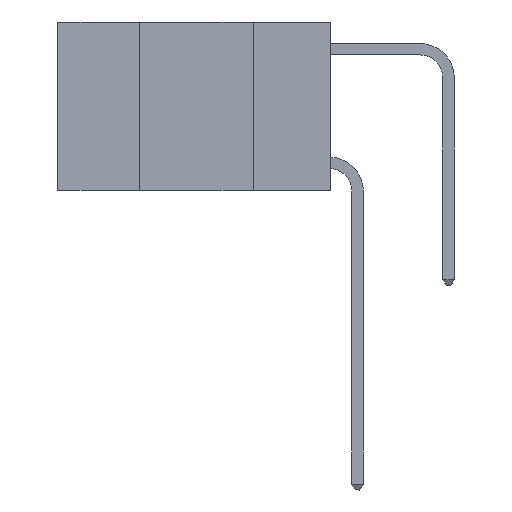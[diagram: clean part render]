
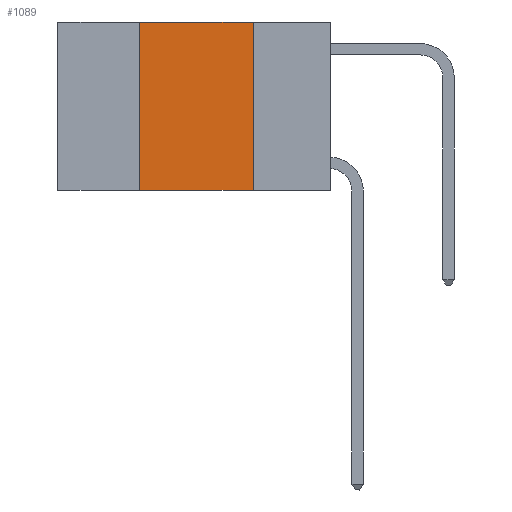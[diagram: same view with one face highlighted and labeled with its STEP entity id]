
A CAD part, left-side view. The second image highlights one B-rep face of the part: STEP entity #1089.
In plain terms, the highlighted planar face has unit normal (-1, 0, 0).
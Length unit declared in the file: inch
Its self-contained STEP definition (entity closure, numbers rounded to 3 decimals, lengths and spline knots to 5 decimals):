
#213 = ORIENTED_EDGE ( 'NONE', *, *, #321, .T. ) ;
#321 = EDGE_CURVE ( 'NONE', #1853, #9964, #543, .T. ) ;
#543 = LINE ( 'NONE', #3451, #1395 ) ;
#1089 = ADVANCED_FACE ( 'NONE', ( #7587 ), #8165, .F. ) ;
#1395 = VECTOR ( 'NONE', #6574, 39.37008 ) ;
#1527 = DIRECTION ( 'NONE',  ( 0., 0., 1. ) ) ;
#1853 = VERTEX_POINT ( 'NONE', #8191 ) ;
#2200 = CARTESIAN_POINT ( 'NONE',  ( 0., 0.17, -0.37 ) ) ;
#2410 = ORIENTED_EDGE ( 'NONE', *, *, #8589, .F. ) ;
#2788 = DIRECTION ( 'NONE',  ( 0., 0., -1. ) ) ;
#2825 = LINE ( 'NONE', #2856, #6476 ) ;
#2856 = CARTESIAN_POINT ( 'NONE',  ( 0., 0.17, 0. ) ) ;
#3275 = CARTESIAN_POINT ( 'NONE',  ( 0., 0.6, 0. ) ) ;
#3351 = DIRECTION ( 'NONE',  ( 0., 0., -1. ) ) ;
#3374 = LINE ( 'NONE', #3275, #10095 ) ;
#3451 = CARTESIAN_POINT ( 'NONE',  ( 0., 0.6, -0.37 ) ) ;
#3969 = CARTESIAN_POINT ( 'NONE',  ( 0., 0.42, 0. ) ) ;
#4024 = EDGE_CURVE ( 'NONE', #6441, #4713, #3374, .T. ) ;
#4118 = CARTESIAN_POINT ( 'NONE',  ( 0., 0.6, 0. ) ) ;
#4713 = VERTEX_POINT ( 'NONE', #8555 ) ;
#4841 = AXIS2_PLACEMENT_3D ( 'NONE', #4118, #4955, #3351 ) ;
#4892 = VECTOR ( 'NONE', #1527, 39.37008 ) ;
#4939 = DIRECTION ( 'NONE',  ( 0., -1., 0. ) ) ;
#4955 = DIRECTION ( 'NONE',  ( 1., 0., 0. ) ) ;
#5157 = CARTESIAN_POINT ( 'NONE',  ( 0., 0.42, 0. ) ) ;
#6441 = VERTEX_POINT ( 'NONE', #3969 ) ;
#6476 = VECTOR ( 'NONE', #2788, 39.37008 ) ;
#6574 = DIRECTION ( 'NONE',  ( 0., -1., 0. ) ) ;
#7587 = FACE_OUTER_BOUND ( 'NONE', #8770, .T. ) ;
#7817 = LINE ( 'NONE', #5157, #4892 ) ;
#8165 = PLANE ( 'NONE',  #4841 ) ;
#8191 = CARTESIAN_POINT ( 'NONE',  ( 0., 0.42, -0.37 ) ) ;
#8415 = ORIENTED_EDGE ( 'NONE', *, *, #4024, .F. ) ;
#8555 = CARTESIAN_POINT ( 'NONE',  ( 0., 0.17, 0. ) ) ;
#8571 = EDGE_CURVE ( 'NONE', #4713, #9964, #2825, .T. ) ;
#8589 = EDGE_CURVE ( 'NONE', #1853, #6441, #7817, .T. ) ;
#8770 = EDGE_LOOP ( 'NONE', ( #9108, #8415, #2410, #213 ) ) ;
#9108 = ORIENTED_EDGE ( 'NONE', *, *, #8571, .F. ) ;
#9964 = VERTEX_POINT ( 'NONE', #2200 ) ;
#10095 = VECTOR ( 'NONE', #4939, 39.37008 ) ;
